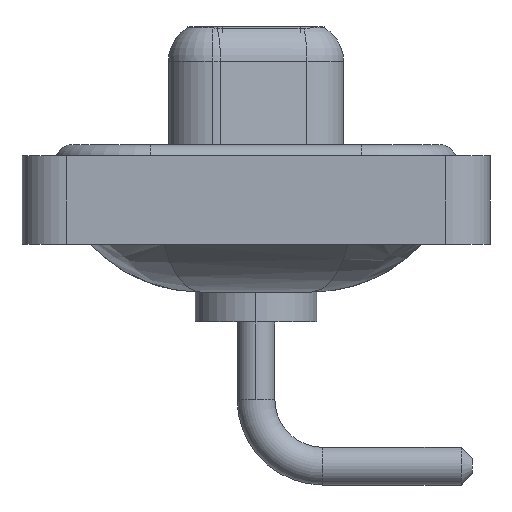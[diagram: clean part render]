
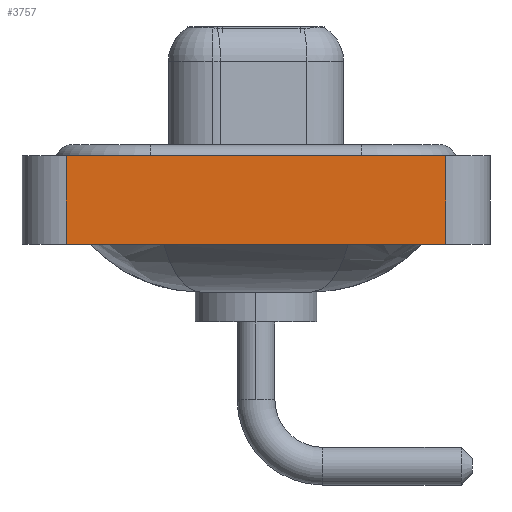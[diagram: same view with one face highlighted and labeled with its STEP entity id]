
A CAD part, left-side view. The second image highlights one B-rep face of the part: STEP entity #3757.
In plain terms, the highlighted planar face has unit normal (-1, 0, 0).
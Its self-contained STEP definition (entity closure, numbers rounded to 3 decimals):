
#994 = CARTESIAN_POINT ( 'NONE',  ( -7.35, 8.55, -3.6 ) ) ;
#1703 = CARTESIAN_POINT ( 'NONE',  ( -7.35, -8.55, 0.4 ) ) ;
#1815 = FACE_OUTER_BOUND ( 'NONE', #4919, .T. ) ;
#1957 = VECTOR ( 'NONE', #4936, 1000. ) ;
#1985 = CARTESIAN_POINT ( 'NONE',  ( -7.35, 8.55, 0.4 ) ) ;
#2200 = DIRECTION ( 'NONE',  ( 0., 0., 1. ) ) ;
#2205 = ORIENTED_EDGE ( 'NONE', *, *, #13822, .F. ) ;
#2283 = LINE ( 'NONE', #7373, #3011 ) ;
#2848 = VERTEX_POINT ( 'NONE', #1703 ) ;
#3011 = VECTOR ( 'NONE', #2200, 1000. ) ;
#3166 = DIRECTION ( 'NONE',  ( 0., 0., 1. ) ) ;
#3540 = VERTEX_POINT ( 'NONE', #14157 ) ;
#3550 = ORIENTED_EDGE ( 'NONE', *, *, #8576, .T. ) ;
#3675 = ORIENTED_EDGE ( 'NONE', *, *, #15690, .F. ) ;
#3757 = ADVANCED_FACE ( 'NONE', ( #1815 ), #6721, .T. ) ;
#4487 = DIRECTION ( 'NONE',  ( -1., 0., 0. ) ) ;
#4919 = EDGE_LOOP ( 'NONE', ( #10156, #3675, #2205, #3550 ) ) ;
#4936 = DIRECTION ( 'NONE',  ( 0., -1., 0. ) ) ;
#5941 = CARTESIAN_POINT ( 'NONE',  ( -7.35, 8.55, -3.6 ) ) ;
#6278 = CARTESIAN_POINT ( 'NONE',  ( -7.35, -8.55, 0.4 ) ) ;
#6721 = PLANE ( 'NONE',  #10353 ) ;
#7321 = LINE ( 'NONE', #994, #13969 ) ;
#7373 = CARTESIAN_POINT ( 'NONE',  ( -7.35, -8.55, -3.6 ) ) ;
#8576 = EDGE_CURVE ( 'NONE', #14242, #3540, #11180, .T. ) ;
#9794 = DIRECTION ( 'NONE',  ( 0., -1., 0. ) ) ;
#10156 = ORIENTED_EDGE ( 'NONE', *, *, #15635, .T. ) ;
#10353 = AXIS2_PLACEMENT_3D ( 'NONE', #15565, #4487, #3166 ) ;
#10979 = DIRECTION ( 'NONE',  ( 0., 0., 1. ) ) ;
#11180 = LINE ( 'NONE', #16336, #1957 ) ;
#12610 = LINE ( 'NONE', #6278, #13370 ) ;
#13370 = VECTOR ( 'NONE', #9794, 1000. ) ;
#13794 = VERTEX_POINT ( 'NONE', #1985 ) ;
#13822 = EDGE_CURVE ( 'NONE', #14242, #13794, #7321, .T. ) ;
#13969 = VECTOR ( 'NONE', #10979, 1000. ) ;
#14157 = CARTESIAN_POINT ( 'NONE',  ( -7.35, -8.55, -3.6 ) ) ;
#14242 = VERTEX_POINT ( 'NONE', #5941 ) ;
#15565 = CARTESIAN_POINT ( 'NONE',  ( -7.35, -8.55, -3.6 ) ) ;
#15635 = EDGE_CURVE ( 'NONE', #3540, #2848, #2283, .T. ) ;
#15690 = EDGE_CURVE ( 'NONE', #13794, #2848, #12610, .T. ) ;
#16336 = CARTESIAN_POINT ( 'NONE',  ( -7.35, -8.55, -3.6 ) ) ;
